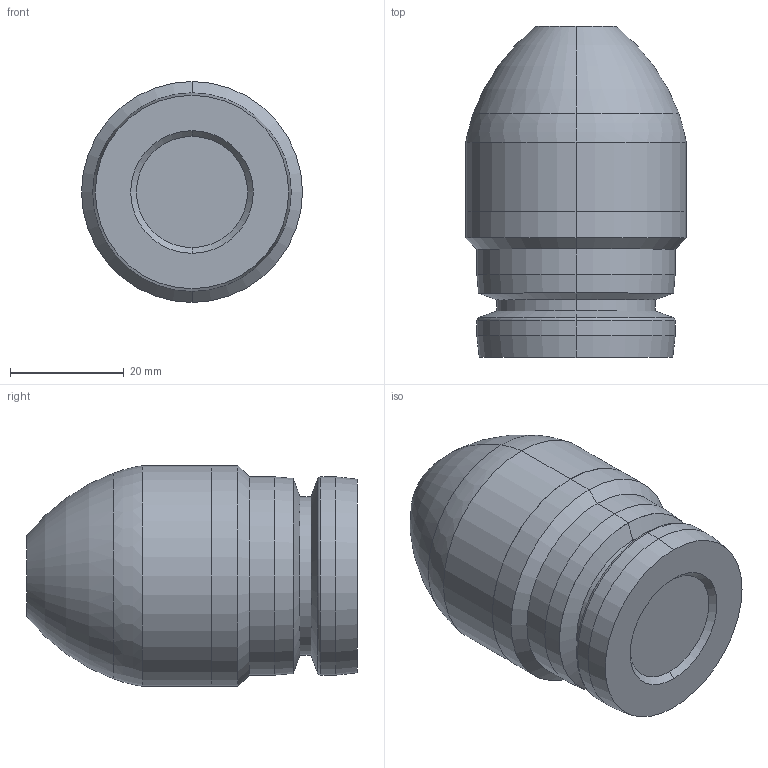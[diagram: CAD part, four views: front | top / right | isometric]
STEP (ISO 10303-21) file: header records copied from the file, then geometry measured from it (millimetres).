
FILE_DESCRIPTION (( 'STEP AP203' ), '1' );
FILE_NAME ('main thin v3.STEP', '2021-12-11T10:36:27', ( '' ), ( '' ), 'SwSTEP 2.0', 'SolidWorks 2020', '' );
FILE_SCHEMA (( 'CONFIG_CONTROL_DESIGN' ));
Length unit declared in the file: inch
Products named in the file (1): main thin v3
Bounding box: 38.86 x 58.21 x 38.86 mm (x, y, z)
Volume: 20678.5 mm3; surface area: 13068.7 mm2
Topology: 1 solids, 1 shells, 50 faces, 98 edges, 56 vertices
Faces by surface type: cone 18, cylinder 12, torus 12, plane 8
Entity records: 1365 total; most frequent: DIRECTION 268, CARTESIAN_POINT 205, ORIENTED_EDGE 196, AXIS2_PLACEMENT_3D 119, EDGE_CURVE 98, CIRCLE 68, VERTEX_POINT 56, EDGE_LOOP 56
